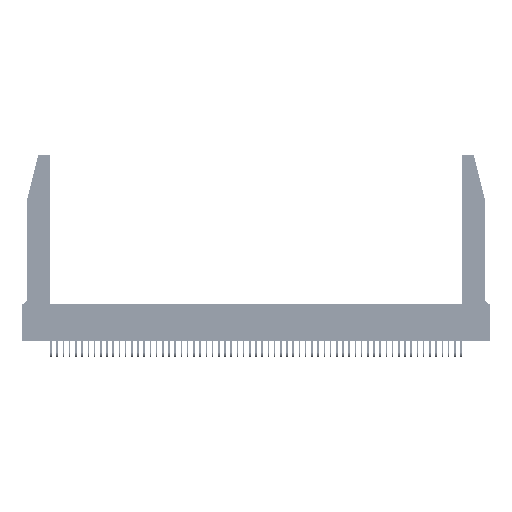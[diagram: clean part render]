
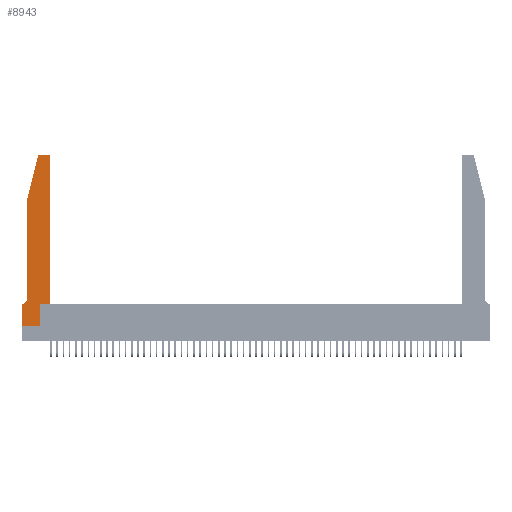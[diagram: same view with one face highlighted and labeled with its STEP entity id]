
A CAD part, top view. The second image highlights one B-rep face of the part: STEP entity #8943.
In plain terms, the highlighted planar face has unit normal (0, 0, 1).
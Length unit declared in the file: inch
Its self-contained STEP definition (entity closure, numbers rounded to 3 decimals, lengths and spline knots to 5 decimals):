
#1156 = CARTESIAN_POINT ( 'NONE',  ( 0.4505, 2.72, 0.37 ) ) ;
#1351 = EDGE_LOOP ( 'NONE', ( #45354, #43494, #19330, #9083, #22092, #5957, #53882, #55452, #25686, #17101, #15831, #29380 ) ) ;
#2642 = EDGE_CURVE ( 'NONE', #52370, #6470, #22050, .T. ) ;
#4281 = DIRECTION ( 'NONE',  ( 1., 0., 0. ) ) ;
#4350 = CIRCLE ( 'NONE', #50965, 0.07 ) ;
#4545 = DIRECTION ( 'NONE',  ( -1., 0., 0. ) ) ;
#5143 = CARTESIAN_POINT ( 'NONE',  ( 0., 0., 0.37 ) ) ;
#5957 = ORIENTED_EDGE ( 'NONE', *, *, #50520, .T. ) ;
#6097 = EDGE_CURVE ( 'NONE', #51687, #24439, #9585, .T. ) ;
#6345 = CARTESIAN_POINT ( 'NONE',  ( 0., 0., 0.37 ) ) ;
#6470 = VERTEX_POINT ( 'NONE', #42588 ) ;
#6933 = CARTESIAN_POINT ( 'NONE',  ( 0., 0., 0.37 ) ) ;
#8224 = VECTOR ( 'NONE', #32207, 39.37008 ) ;
#8233 = DIRECTION ( 'NONE',  ( -1., 0., 0. ) ) ;
#8852 = DIRECTION ( 'NONE',  ( 0., 0., -1. ) ) ;
#8943 = ADVANCED_FACE ( 'NONE', ( #53251 ), #11861, .T. ) ;
#9083 = ORIENTED_EDGE ( 'NONE', *, *, #2642, .T. ) ;
#9585 = LINE ( 'NONE', #18615, #53967 ) ;
#9893 = AXIS2_PLACEMENT_3D ( 'NONE', #29455, #16571, #12050 ) ;
#9978 = DIRECTION ( 'NONE',  ( 0., 1., 0. ) ) ;
#10527 = DIRECTION ( 'NONE',  ( 1., 0., 0. ) ) ;
#10955 = CARTESIAN_POINT ( 'NONE',  ( 0.4205, 2.75, 0.37 ) ) ;
#11156 = EDGE_CURVE ( 'NONE', #32487, #51601, #24659, .T. ) ;
#11761 = DIRECTION ( 'NONE',  ( 0., 1., 0. ) ) ;
#11861 = PLANE ( 'NONE',  #9893 ) ;
#11989 = EDGE_CURVE ( 'NONE', #54615, #24963, #28709, .T. ) ;
#12050 = DIRECTION ( 'NONE',  ( 1., 0., 0. ) ) ;
#12415 = CARTESIAN_POINT ( 'NONE',  ( 0.2865, 0., 0.37 ) ) ;
#12463 = CARTESIAN_POINT ( 'NONE',  ( 0.284, 2.75, 0.37 ) ) ;
#13623 = LINE ( 'NONE', #6345, #8224 ) ;
#14563 = EDGE_CURVE ( 'NONE', #51601, #47431, #50250, .T. ) ;
#15418 = VERTEX_POINT ( 'NONE', #41694 ) ;
#15831 = ORIENTED_EDGE ( 'NONE', *, *, #16457, .T. ) ;
#16457 = EDGE_CURVE ( 'NONE', #36568, #32487, #38564, .T. ) ;
#16571 = DIRECTION ( 'NONE',  ( 0., 0., 1. ) ) ;
#16646 = CARTESIAN_POINT ( 'NONE',  ( 0.2605, 2.75, 0.37 ) ) ;
#17101 = ORIENTED_EDGE ( 'NONE', *, *, #31219, .T. ) ;
#17228 = DIRECTION ( 'NONE',  ( 0., 0., 1. ) ) ;
#17970 = VECTOR ( 'NONE', #46281, 39.37008 ) ;
#18508 = EDGE_CURVE ( 'NONE', #47431, #34641, #34253, .T. ) ;
#18615 = CARTESIAN_POINT ( 'NONE',  ( 0.2865, 0.35, 0.37 ) ) ;
#18724 = CARTESIAN_POINT ( 'NONE',  ( 0.2865, 0.35, 0.37 ) ) ;
#19057 = VECTOR ( 'NONE', #8233, 39.37008 ) ;
#19330 = ORIENTED_EDGE ( 'NONE', *, *, #31136, .T. ) ;
#19548 = VECTOR ( 'NONE', #21511, 39.37008 ) ;
#20234 = EDGE_CURVE ( 'NONE', #6470, #15418, #4350, .T. ) ;
#21155 = EDGE_CURVE ( 'NONE', #24963, #51687, #13623, .T. ) ;
#21511 = DIRECTION ( 'NONE',  ( -0.239, -0.971, 0. ) ) ;
#22050 = LINE ( 'NONE', #32040, #35454 ) ;
#22092 = ORIENTED_EDGE ( 'NONE', *, *, #20234, .T. ) ;
#22867 = AXIS2_PLACEMENT_3D ( 'NONE', #34083, #17228, #4281 ) ;
#23415 = DIRECTION ( 'NONE',  ( 0., -1., 0. ) ) ;
#24439 = VERTEX_POINT ( 'NONE', #18724 ) ;
#24659 = CIRCLE ( 'NONE', #22867, 0.03 ) ;
#24963 = VERTEX_POINT ( 'NONE', #5143 ) ;
#25686 = ORIENTED_EDGE ( 'NONE', *, *, #6097, .T. ) ;
#28709 = LINE ( 'NONE', #6933, #42078 ) ;
#29380 = ORIENTED_EDGE ( 'NONE', *, *, #11156, .T. ) ;
#29455 = CARTESIAN_POINT ( 'NONE',  ( 0., 0.35, 0.37 ) ) ;
#30915 = LINE ( 'NONE', #47251, #19548 ) ;
#31136 = EDGE_CURVE ( 'NONE', #34641, #52370, #30915, .T. ) ;
#31219 = EDGE_CURVE ( 'NONE', #24439, #36568, #46353, .T. ) ;
#31717 = CARTESIAN_POINT ( 'NONE',  ( 0.284, 2.72, 0.37 ) ) ;
#32040 = CARTESIAN_POINT ( 'NONE',  ( 0.0755, 2., 0.37 ) ) ;
#32207 = DIRECTION ( 'NONE',  ( 1., 0., 0. ) ) ;
#32487 = VERTEX_POINT ( 'NONE', #1156 ) ;
#32536 = VECTOR ( 'NONE', #11761, 39.37008 ) ;
#33913 = CARTESIAN_POINT ( 'NONE',  ( 0.0755, 0.35, 0.37 ) ) ;
#34058 = CARTESIAN_POINT ( 'NONE',  ( 0.4505, 0.35, 0.37 ) ) ;
#34083 = CARTESIAN_POINT ( 'NONE',  ( 0.4205, 2.72, 0.37 ) ) ;
#34253 = CIRCLE ( 'NONE', #50892, 0.03 ) ;
#34641 = VERTEX_POINT ( 'NONE', #42006 ) ;
#35454 = VECTOR ( 'NONE', #23415, 39.37008 ) ;
#36214 = DIRECTION ( 'NONE',  ( 0., 0., 1. ) ) ;
#36568 = VERTEX_POINT ( 'NONE', #49944 ) ;
#37293 = DIRECTION ( 'NONE',  ( 0., -1., 0. ) ) ;
#38564 = LINE ( 'NONE', #45738, #32536 ) ;
#39416 = CARTESIAN_POINT ( 'NONE',  ( 0.0055, 0.42, 0.37 ) ) ;
#39803 = LINE ( 'NONE', #33913, #19057 ) ;
#41193 = CARTESIAN_POINT ( 'NONE',  ( 0.0755, 2., 0.37 ) ) ;
#41694 = CARTESIAN_POINT ( 'NONE',  ( 0.0055, 0.35, 0.37 ) ) ;
#42006 = CARTESIAN_POINT ( 'NONE',  ( 0.25487, 2.72718, 0.37 ) ) ;
#42078 = VECTOR ( 'NONE', #37293, 39.37008 ) ;
#42588 = CARTESIAN_POINT ( 'NONE',  ( 0.0755, 0.42, 0.37 ) ) ;
#43494 = ORIENTED_EDGE ( 'NONE', *, *, #18508, .T. ) ;
#45354 = ORIENTED_EDGE ( 'NONE', *, *, #14563, .T. ) ;
#45647 = VECTOR ( 'NONE', #52716, 39.37008 ) ;
#45738 = CARTESIAN_POINT ( 'NONE',  ( 0.4505, 0.35, 0.37 ) ) ;
#46281 = DIRECTION ( 'NONE',  ( -1., 0., 0. ) ) ;
#46353 = LINE ( 'NONE', #34058, #45647 ) ;
#47251 = CARTESIAN_POINT ( 'NONE',  ( 0.0755, 2., 0.37 ) ) ;
#47431 = VERTEX_POINT ( 'NONE', #12463 ) ;
#47952 = CARTESIAN_POINT ( 'NONE',  ( 0., 0.35, 0.37 ) ) ;
#49944 = CARTESIAN_POINT ( 'NONE',  ( 0.4505, 0.35, 0.37 ) ) ;
#50250 = LINE ( 'NONE', #16646, #17970 ) ;
#50520 = EDGE_CURVE ( 'NONE', #15418, #54615, #39803, .T. ) ;
#50892 = AXIS2_PLACEMENT_3D ( 'NONE', #31717, #36214, #10527 ) ;
#50965 = AXIS2_PLACEMENT_3D ( 'NONE', #39416, #8852, #4545 ) ;
#51601 = VERTEX_POINT ( 'NONE', #10955 ) ;
#51687 = VERTEX_POINT ( 'NONE', #12415 ) ;
#52370 = VERTEX_POINT ( 'NONE', #41193 ) ;
#52716 = DIRECTION ( 'NONE',  ( 1., 0., 0. ) ) ;
#53251 = FACE_OUTER_BOUND ( 'NONE', #1351, .T. ) ;
#53882 = ORIENTED_EDGE ( 'NONE', *, *, #11989, .T. ) ;
#53967 = VECTOR ( 'NONE', #9978, 39.37008 ) ;
#54615 = VERTEX_POINT ( 'NONE', #47952 ) ;
#55452 = ORIENTED_EDGE ( 'NONE', *, *, #21155, .T. ) ;
